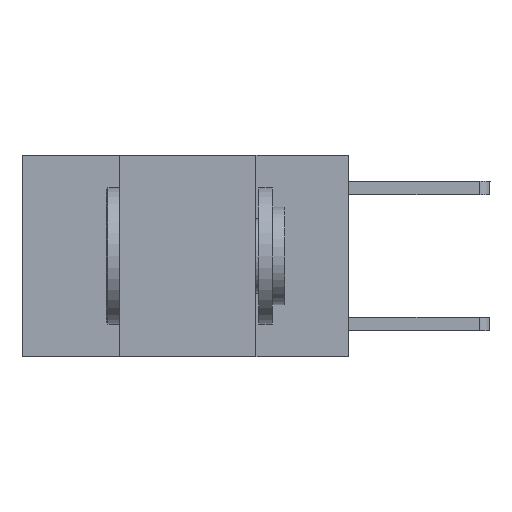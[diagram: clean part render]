
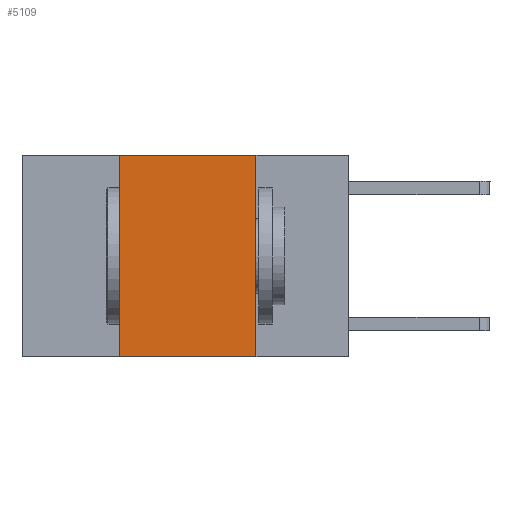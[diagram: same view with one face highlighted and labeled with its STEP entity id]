
A CAD part, left-side view. The second image highlights one B-rep face of the part: STEP entity #5109.
In plain terms, the highlighted planar face has unit normal (-1, 0, 0).
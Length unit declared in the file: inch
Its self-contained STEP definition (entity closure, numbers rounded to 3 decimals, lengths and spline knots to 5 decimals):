
#26 = CARTESIAN_POINT ( 'NONE',  ( 0., 0.6, 0. ) ) ;
#473 = VERTEX_POINT ( 'NONE', #4364 ) ;
#579 = VERTEX_POINT ( 'NONE', #7220 ) ;
#622 = EDGE_CURVE ( 'NONE', #473, #579, #1493, .T. ) ;
#674 = ORIENTED_EDGE ( 'NONE', *, *, #9423, .F. ) ;
#744 = EDGE_CURVE ( 'NONE', #3234, #783, #4088, .T. ) ;
#783 = VERTEX_POINT ( 'NONE', #6486 ) ;
#1493 = LINE ( 'NONE', #10204, #9599 ) ;
#1802 = EDGE_CURVE ( 'NONE', #783, #579, #8971, .T. ) ;
#1947 = VECTOR ( 'NONE', #3249, 39.37008 ) ;
#2078 = PLANE ( 'NONE',  #7551 ) ;
#2722 = DIRECTION ( 'NONE',  ( 0., 0., -1. ) ) ;
#3234 = VERTEX_POINT ( 'NONE', #9651 ) ;
#3249 = DIRECTION ( 'NONE',  ( 0., -1., 0. ) ) ;
#3781 = DIRECTION ( 'NONE',  ( 0., 0., -1. ) ) ;
#4088 = LINE ( 'NONE', #26, #1947 ) ;
#4364 = CARTESIAN_POINT ( 'NONE',  ( 0., 0.42, -0.37 ) ) ;
#4706 = ORIENTED_EDGE ( 'NONE', *, *, #744, .F. ) ;
#5109 = ADVANCED_FACE ( 'NONE', ( #9214 ), #2078, .F. ) ;
#5117 = CARTESIAN_POINT ( 'NONE',  ( 0., 0.6, 0. ) ) ;
#5212 = DIRECTION ( 'NONE',  ( 1., 0., 0. ) ) ;
#5310 = LINE ( 'NONE', #9360, #5333 ) ;
#5316 = VECTOR ( 'NONE', #3781, 39.37008 ) ;
#5333 = VECTOR ( 'NONE', #9316, 39.37008 ) ;
#5419 = ORIENTED_EDGE ( 'NONE', *, *, #1802, .F. ) ;
#6486 = CARTESIAN_POINT ( 'NONE',  ( 0., 0.17, 0. ) ) ;
#7220 = CARTESIAN_POINT ( 'NONE',  ( 0., 0.17, -0.37 ) ) ;
#7551 = AXIS2_PLACEMENT_3D ( 'NONE', #5117, #5212, #2722 ) ;
#8773 = ORIENTED_EDGE ( 'NONE', *, *, #622, .T. ) ;
#8918 = CARTESIAN_POINT ( 'NONE',  ( 0., 0.17, 0. ) ) ;
#8971 = LINE ( 'NONE', #8918, #5316 ) ;
#9214 = FACE_OUTER_BOUND ( 'NONE', #9751, .T. ) ;
#9316 = DIRECTION ( 'NONE',  ( 0., 0., 1. ) ) ;
#9360 = CARTESIAN_POINT ( 'NONE',  ( 0., 0.42, 0. ) ) ;
#9423 = EDGE_CURVE ( 'NONE', #473, #3234, #5310, .T. ) ;
#9599 = VECTOR ( 'NONE', #10311, 39.37008 ) ;
#9651 = CARTESIAN_POINT ( 'NONE',  ( 0., 0.42, 0. ) ) ;
#9751 = EDGE_LOOP ( 'NONE', ( #5419, #4706, #674, #8773 ) ) ;
#10204 = CARTESIAN_POINT ( 'NONE',  ( 0., 0.6, -0.37 ) ) ;
#10311 = DIRECTION ( 'NONE',  ( 0., -1., 0. ) ) ;
